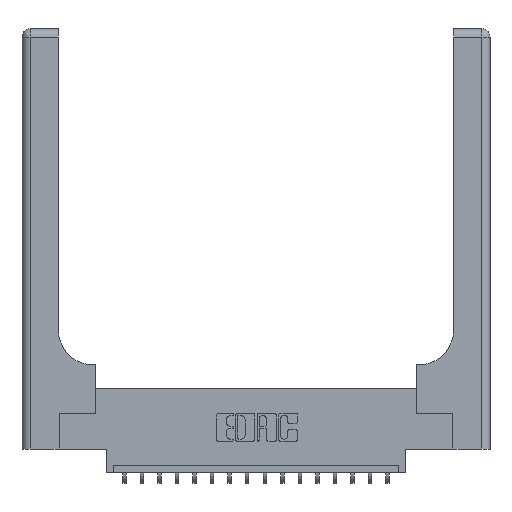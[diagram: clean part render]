
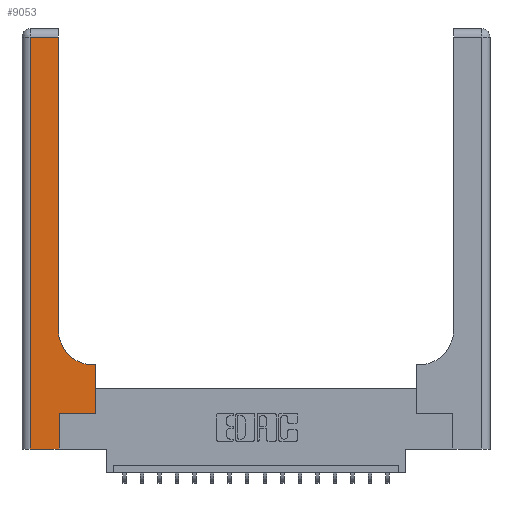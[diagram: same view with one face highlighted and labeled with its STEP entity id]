
A CAD part, top view. The second image highlights one B-rep face of the part: STEP entity #9053.
In plain terms, the highlighted planar face has unit normal (0, 0, 1).
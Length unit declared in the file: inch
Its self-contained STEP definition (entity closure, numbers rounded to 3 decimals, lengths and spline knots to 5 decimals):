
#65 = DIRECTION ( 'NONE',  ( 0., 1., 0. ) ) ;
#162 = DIRECTION ( 'NONE',  ( 1., 0., 0. ) ) ;
#307 = CARTESIAN_POINT ( 'NONE',  ( 0.528, 0.25, 0.37 ) ) ;
#351 = CARTESIAN_POINT ( 'NONE',  ( 0.51, 0.6, 0.37 ) ) ;
#526 = CARTESIAN_POINT ( 'NONE',  ( 0., 0., 0.37 ) ) ;
#561 = VECTOR ( 'NONE', #15979, 39.37008 ) ;
#1587 = VECTOR ( 'NONE', #65, 39.37008 ) ;
#1761 = LINE ( 'NONE', #10788, #2698 ) ;
#2165 = ORIENTED_EDGE ( 'NONE', *, *, #13721, .T. ) ;
#2292 = CIRCLE ( 'NONE', #18068, 0.25 ) ;
#2318 = VERTEX_POINT ( 'NONE', #16621 ) ;
#2621 = VECTOR ( 'NONE', #8471, 39.37008 ) ;
#2698 = VECTOR ( 'NONE', #13703, 39.37008 ) ;
#2933 = CARTESIAN_POINT ( 'NONE',  ( 0.26, 3., 0.37 ) ) ;
#3175 = CARTESIAN_POINT ( 'NONE',  ( 0.265, 0., 0.37 ) ) ;
#3307 = DIRECTION ( 'NONE',  ( 0., 0., -1. ) ) ;
#3807 = CARTESIAN_POINT ( 'NONE',  ( 0.265, 0.25, 0.37 ) ) ;
#3810 = CARTESIAN_POINT ( 'NONE',  ( 0.265, 0., 0.37 ) ) ;
#4122 = DIRECTION ( 'NONE',  ( 0., 0., -1. ) ) ;
#4127 = VERTEX_POINT ( 'NONE', #307 ) ;
#4319 = VERTEX_POINT ( 'NONE', #3807 ) ;
#4459 = EDGE_CURVE ( 'NONE', #6280, #12807, #2292, .T. ) ;
#4732 = VERTEX_POINT ( 'NONE', #14775 ) ;
#5405 = LINE ( 'NONE', #17587, #16545 ) ;
#5781 = CARTESIAN_POINT ( 'NONE',  ( 0., 2.94, 0.37 ) ) ;
#6172 = EDGE_CURVE ( 'NONE', #4319, #4127, #5405, .T. ) ;
#6280 = VERTEX_POINT ( 'NONE', #351 ) ;
#6373 = DIRECTION ( 'NONE',  ( 1., 0., 0. ) ) ;
#6398 = EDGE_CURVE ( 'NONE', #4732, #12350, #1761, .T. ) ;
#6700 = ORIENTED_EDGE ( 'NONE', *, *, #7391, .T. ) ;
#7174 = ORIENTED_EDGE ( 'NONE', *, *, #6398, .T. ) ;
#7391 = EDGE_CURVE ( 'NONE', #13872, #4732, #10602, .T. ) ;
#7894 = CARTESIAN_POINT ( 'NONE',  ( 0.06, 0., 0.37 ) ) ;
#8000 = EDGE_CURVE ( 'NONE', #12807, #13872, #13091, .T. ) ;
#8085 = ORIENTED_EDGE ( 'NONE', *, *, #9581, .T. ) ;
#8471 = DIRECTION ( 'NONE',  ( -1., 0., 0. ) ) ;
#8908 = CARTESIAN_POINT ( 'NONE',  ( 0.26, 2.94, 0.37 ) ) ;
#8995 = ORIENTED_EDGE ( 'NONE', *, *, #6172, .T. ) ;
#9053 = ADVANCED_FACE ( 'NONE', ( #18743 ), #9070, .F. ) ;
#9070 = PLANE ( 'NONE',  #18665 ) ;
#9581 = EDGE_CURVE ( 'NONE', #17385, #4319, #17258, .T. ) ;
#9874 = LINE ( 'NONE', #17158, #2621 ) ;
#10258 = EDGE_LOOP ( 'NONE', ( #13969, #6700, #7174, #18751, #8085, #8995, #13323, #2165, #14220 ) ) ;
#10602 = LINE ( 'NONE', #5781, #11053 ) ;
#10788 = CARTESIAN_POINT ( 'NONE',  ( 0.06, 3., 0.37 ) ) ;
#10942 = VECTOR ( 'NONE', #6373, 39.37008 ) ;
#11053 = VECTOR ( 'NONE', #14481, 39.37008 ) ;
#11921 = DIRECTION ( 'NONE',  ( 0., 1., 0. ) ) ;
#12350 = VERTEX_POINT ( 'NONE', #7894 ) ;
#12728 = LINE ( 'NONE', #16006, #1587 ) ;
#12807 = VERTEX_POINT ( 'NONE', #16503 ) ;
#12819 = CARTESIAN_POINT ( 'NONE',  ( 0.51, 0.85, 0.37 ) ) ;
#13091 = LINE ( 'NONE', #2933, #561 ) ;
#13323 = ORIENTED_EDGE ( 'NONE', *, *, #18697, .T. ) ;
#13391 = CARTESIAN_POINT ( 'NONE',  ( 0., 3., 0.37 ) ) ;
#13411 = VECTOR ( 'NONE', #11921, 39.37008 ) ;
#13464 = DIRECTION ( 'NONE',  ( -1., 0., 0. ) ) ;
#13703 = DIRECTION ( 'NONE',  ( 0., -1., 0. ) ) ;
#13721 = EDGE_CURVE ( 'NONE', #2318, #6280, #9874, .T. ) ;
#13872 = VERTEX_POINT ( 'NONE', #8908 ) ;
#13969 = ORIENTED_EDGE ( 'NONE', *, *, #8000, .T. ) ;
#14220 = ORIENTED_EDGE ( 'NONE', *, *, #4459, .T. ) ;
#14276 = DIRECTION ( 'NONE',  ( 1., 0., 0. ) ) ;
#14481 = DIRECTION ( 'NONE',  ( -1., 0., 0. ) ) ;
#14775 = CARTESIAN_POINT ( 'NONE',  ( 0.06, 2.94, 0.37 ) ) ;
#14792 = LINE ( 'NONE', #526, #10942 ) ;
#15979 = DIRECTION ( 'NONE',  ( 0., 1., 0. ) ) ;
#16006 = CARTESIAN_POINT ( 'NONE',  ( 0.528, 0.25, 0.37 ) ) ;
#16503 = CARTESIAN_POINT ( 'NONE',  ( 0.26, 0.85, 0.37 ) ) ;
#16545 = VECTOR ( 'NONE', #162, 39.37008 ) ;
#16621 = CARTESIAN_POINT ( 'NONE',  ( 0.528, 0.6, 0.37 ) ) ;
#17158 = CARTESIAN_POINT ( 'NONE',  ( 0.26, 0.6, 0.37 ) ) ;
#17258 = LINE ( 'NONE', #3175, #13411 ) ;
#17385 = VERTEX_POINT ( 'NONE', #3810 ) ;
#17587 = CARTESIAN_POINT ( 'NONE',  ( 0.265, 0.25, 0.37 ) ) ;
#18068 = AXIS2_PLACEMENT_3D ( 'NONE', #12819, #4122, #14276 ) ;
#18325 = EDGE_CURVE ( 'NONE', #12350, #17385, #14792, .T. ) ;
#18665 = AXIS2_PLACEMENT_3D ( 'NONE', #13391, #3307, #13464 ) ;
#18697 = EDGE_CURVE ( 'NONE', #4127, #2318, #12728, .T. ) ;
#18743 = FACE_OUTER_BOUND ( 'NONE', #10258, .T. ) ;
#18751 = ORIENTED_EDGE ( 'NONE', *, *, #18325, .T. ) ;
